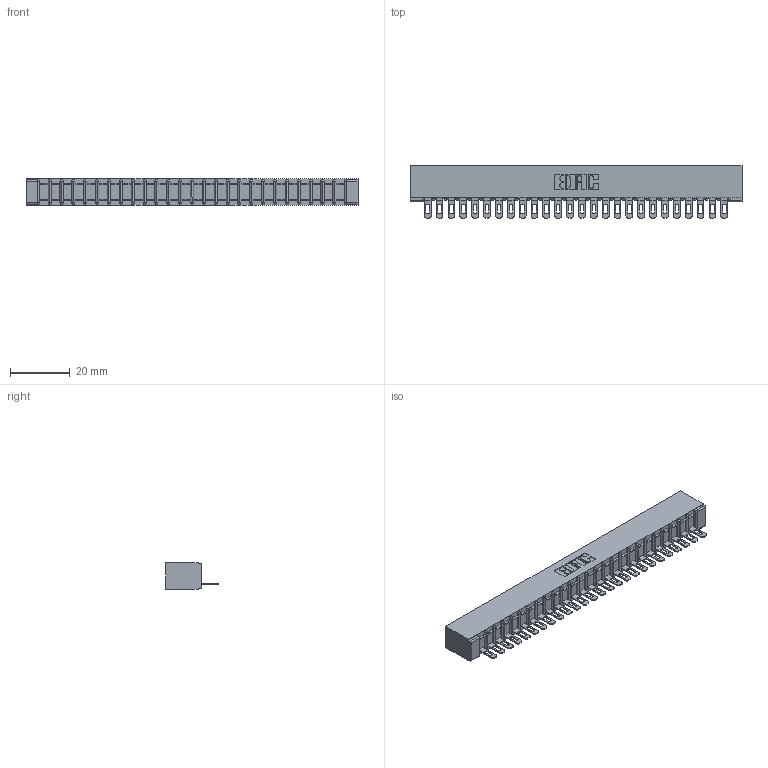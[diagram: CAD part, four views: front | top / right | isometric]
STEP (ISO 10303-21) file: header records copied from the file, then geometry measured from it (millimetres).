
FILE_DESCRIPTION (( 'STEP AP203' ), '1' );
FILE_NAME ('307-026-501-101.STEP', '2018-08-04T13:52:02', ( '' ), ( '' ), 'SwSTEP 2.0', 'SolidWorks 2016', '' );
FILE_SCHEMA (( 'CONFIG_CONTROL_DESIGN' ));
Length unit declared in the file: inch
Products named in the file (3): 307-290-002_501; 307-026-501-101; 307 Part_No Mounting Lugs
Assembly tree (27 placements, depth 2):
  307-026-501-101
    307 Part_No Mounting Lugs
    307-290-002_501  x26
Bounding box: 110.9 x 17.42 x 8.71 mm (x, y, z)
Volume: 7588.2 mm3; surface area: 14706.3 mm2
Topology: 27 solids, 27 shells, 2113 faces, 6487 edges, 4250 vertices
Faces by surface type: plane 1210, cylinder 849, sphere 54
Entity records: 24778 total; most frequent: CARTESIAN_POINT 4176, ORIENTED_EDGE 4166, DIRECTION 4067, EDGE_CURVE 2083, LINE 1585, VECTOR 1585, VERTEX_POINT 1350, AXIS2_PLACEMENT_3D 1241
